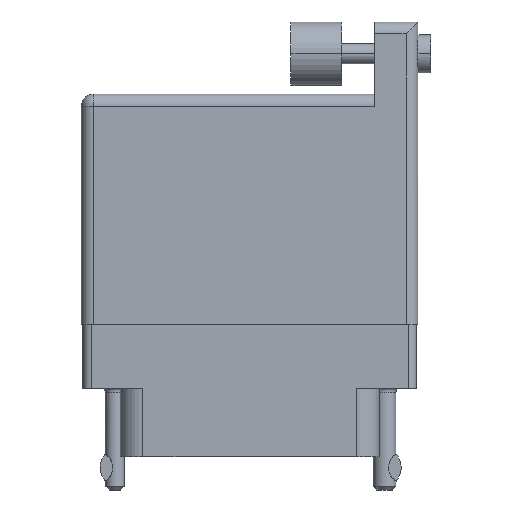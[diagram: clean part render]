
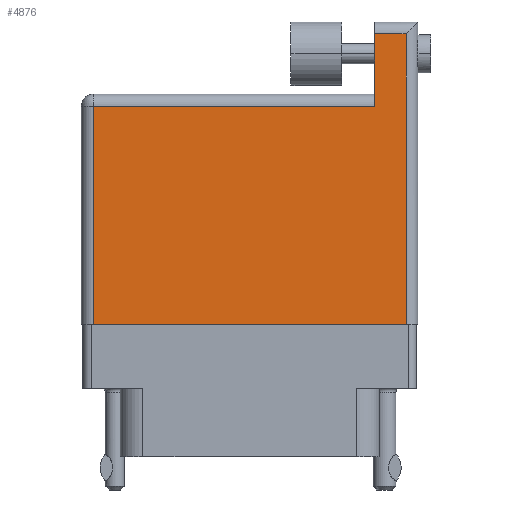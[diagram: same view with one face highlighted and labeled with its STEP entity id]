
A CAD part, front view. The second image highlights one B-rep face of the part: STEP entity #4876.
In plain terms, the highlighted face is planar.
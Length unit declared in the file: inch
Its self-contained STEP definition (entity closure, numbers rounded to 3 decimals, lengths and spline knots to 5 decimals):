
#406 = EDGE_CURVE ( 'NONE', #3256, #30625, #16142, .T. ) ;
#1185 = DIRECTION ( 'NONE',  ( -1., 0., 0. ) ) ;
#1224 = CARTESIAN_POINT ( 'NONE',  ( 1.278, 1.143, 0. ) ) ;
#1835 = ORIENTED_EDGE ( 'NONE', *, *, #18360, .T. ) ;
#1884 = LINE ( 'NONE', #29521, #19166 ) ;
#2318 = DIRECTION ( 'NONE',  ( 0., 0., -1. ) ) ;
#3256 = VERTEX_POINT ( 'NONE', #16449 ) ;
#4226 = ORIENTED_EDGE ( 'NONE', *, *, #406, .T. ) ;
#4876 = ADVANCED_FACE ( 'NONE', ( #10829 ), #15918, .F. ) ;
#5509 = ORIENTED_EDGE ( 'NONE', *, *, #34148, .T. ) ;
#6638 = EDGE_CURVE ( 'NONE', #18581, #34897, #22795, .T. ) ;
#6836 = CARTESIAN_POINT ( 'NONE',  ( 1.155, 1.143, 0. ) ) ;
#6958 = CARTESIAN_POINT ( 'NONE',  ( 0., 0.859, 0. ) ) ;
#7179 = VECTOR ( 'NONE', #1185, 39.37008 ) ;
#7979 = CARTESIAN_POINT ( 'NONE',  ( 0., 0.906, 0. ) ) ;
#8760 = DIRECTION ( 'NONE',  ( 0., -1., 0. ) ) ;
#8998 = VECTOR ( 'NONE', #18986, 39.37008 ) ;
#9618 = VECTOR ( 'NONE', #8760, 39.37008 ) ;
#10829 = FACE_OUTER_BOUND ( 'NONE', #17065, .T. ) ;
#10892 = ORIENTED_EDGE ( 'NONE', *, *, #11101, .T. ) ;
#11101 = EDGE_CURVE ( 'NONE', #30625, #17763, #1884, .T. ) ;
#12197 = AXIS2_PLACEMENT_3D ( 'NONE', #7979, #2318, #13526 ) ;
#13066 = DIRECTION ( 'NONE',  ( 0., 1., 0. ) ) ;
#13526 = DIRECTION ( 'NONE',  ( -1., 0., 0. ) ) ;
#14697 = VERTEX_POINT ( 'NONE', #35316 ) ;
#15639 = ORIENTED_EDGE ( 'NONE', *, *, #24968, .T. ) ;
#15813 = LINE ( 'NONE', #6958, #7179 ) ;
#15918 = PLANE ( 'NONE',  #12197 ) ;
#16142 = LINE ( 'NONE', #28402, #20443 ) ;
#16449 = CARTESIAN_POINT ( 'NONE',  ( 0.047, 0., 0. ) ) ;
#16641 = CARTESIAN_POINT ( 'NONE',  ( 1.155, 1.19, 0. ) ) ;
#17065 = EDGE_LOOP ( 'NONE', ( #4226, #10892, #1835, #21641, #5509, #15639 ) ) ;
#17206 = CARTESIAN_POINT ( 'NONE',  ( 1.155, 1.143, 0. ) ) ;
#17763 = VERTEX_POINT ( 'NONE', #1224 ) ;
#18360 = EDGE_CURVE ( 'NONE', #17763, #18581, #33998, .T. ) ;
#18581 = VERTEX_POINT ( 'NONE', #6836 ) ;
#18986 = DIRECTION ( 'NONE',  ( 0., -1., 0. ) ) ;
#19166 = VECTOR ( 'NONE', #13066, 39.37008 ) ;
#20443 = VECTOR ( 'NONE', #23101, 39.37008 ) ;
#21641 = ORIENTED_EDGE ( 'NONE', *, *, #6638, .T. ) ;
#22795 = LINE ( 'NONE', #16641, #8998 ) ;
#23101 = DIRECTION ( 'NONE',  ( 1., 0., 0. ) ) ;
#24968 = EDGE_CURVE ( 'NONE', #14697, #3256, #34169, .T. ) ;
#26074 = CARTESIAN_POINT ( 'NONE',  ( 1.155, 0.859, 0. ) ) ;
#27930 = DIRECTION ( 'NONE',  ( -1., 0., 0. ) ) ;
#28402 = CARTESIAN_POINT ( 'NONE',  ( 0., 0., 0. ) ) ;
#29521 = CARTESIAN_POINT ( 'NONE',  ( 1.278, 1.19, 0. ) ) ;
#29700 = VECTOR ( 'NONE', #27930, 39.37008 ) ;
#30625 = VERTEX_POINT ( 'NONE', #33576 ) ;
#33200 = CARTESIAN_POINT ( 'NONE',  ( 0.047, 0., 0. ) ) ;
#33576 = CARTESIAN_POINT ( 'NONE',  ( 1.278, 0., 0. ) ) ;
#33998 = LINE ( 'NONE', #17206, #29700 ) ;
#34148 = EDGE_CURVE ( 'NONE', #34897, #14697, #15813, .T. ) ;
#34169 = LINE ( 'NONE', #33200, #9618 ) ;
#34897 = VERTEX_POINT ( 'NONE', #26074 ) ;
#35316 = CARTESIAN_POINT ( 'NONE',  ( 0.047, 0.859, 0. ) ) ;
